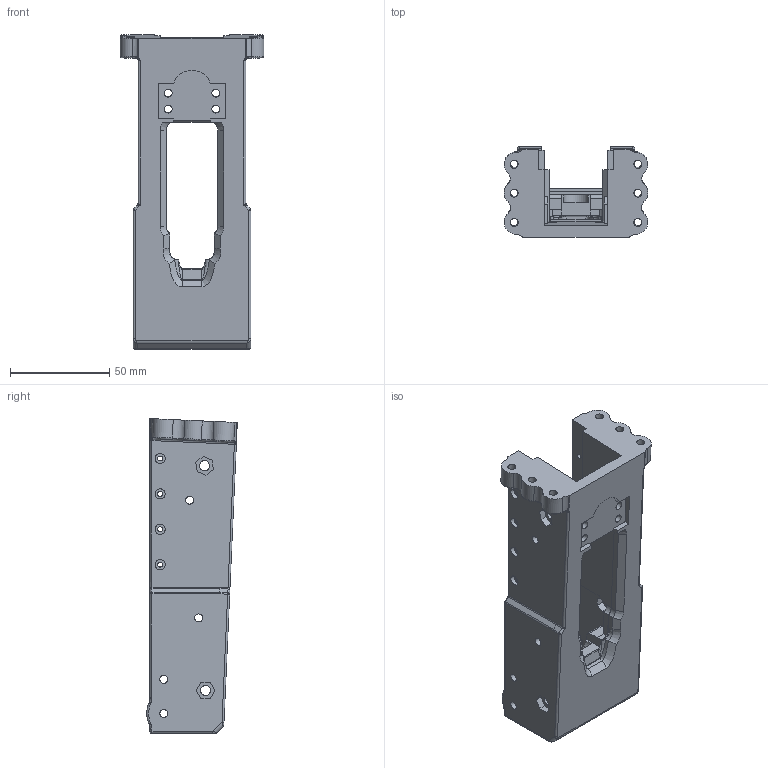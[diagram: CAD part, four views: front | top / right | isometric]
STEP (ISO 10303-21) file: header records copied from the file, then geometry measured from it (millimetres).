
FILE_DESCRIPTION(/* description */ (''),/* implementation_level */ '2;1');
FILE_NAME(/* name */ 'Plastikov v3.0 Standard Front Receiver.stp',/* time_stamp */ '2022-03-22T10:44:58-05:00',/* author */ ('johne'),/* organization */ (''),/* preprocessor_version */ 'ST-DEVELOPER v18.1',/* originating_system */ 'Autodesk Inventor 2020',/* authorisation */ '');
FILE_SCHEMA (('AUTOMOTIVE_DESIGN { 1 0 10303 214 3 1 1 }'));
Length unit declared in the file: millimetre
Products named in the file (1): Plastikov v3.0 Standard Front Receiver
Bounding box: 72.2 x 45.54 x 158.19 mm (x, y, z)
Volume: 184799.2 mm3; surface area: 46767.3 mm2
Topology: 1 solids, 1 shells, 368 faces, 968 edges, 604 vertices
Faces by surface type: plane 168, cylinder 116, bspline 51, torus 18, sphere 9, cone 6
Full cylindrical faces by diameter (mm): 2.5 x8, 4 x18, 5 x1, 5.08 x8, 5.1 x2, 11.989 x1, 12 x1
Entity records: 13092 total; most frequent: CARTESIAN_POINT 3964, ORIENTED_EDGE 1904, DIRECTION 1848, EDGE_CURVE 952, AXIS2_PLACEMENT_3D 650, VERTEX_POINT 604, LINE 548, VECTOR 548
